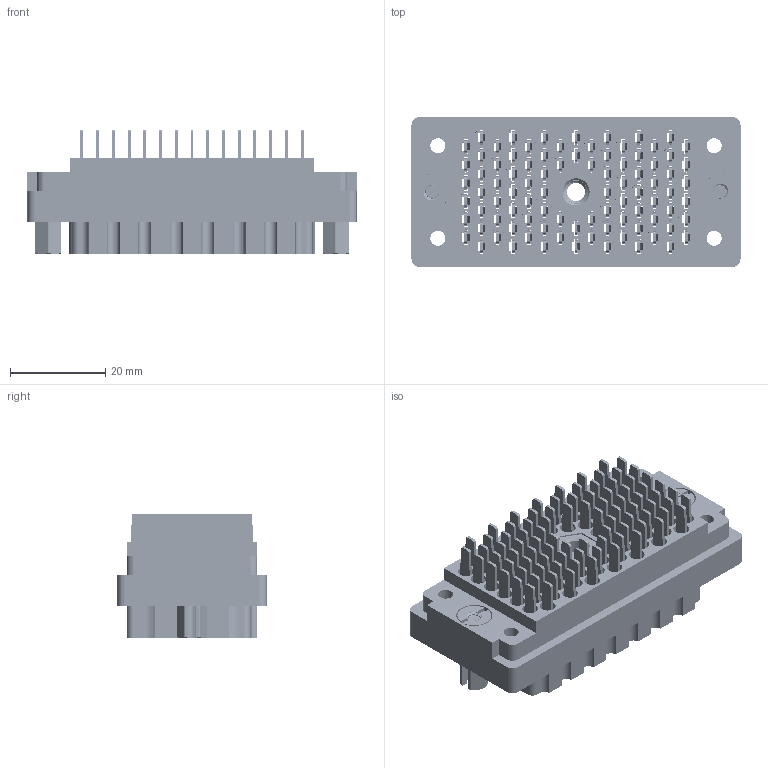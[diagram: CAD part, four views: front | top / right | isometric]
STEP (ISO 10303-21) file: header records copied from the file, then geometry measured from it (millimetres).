
FILE_DESCRIPTION (( 'STEP AP203' ), '1' );
FILE_NAME ('516-090-501-202.STEP', '2020-09-08T17:35:47', ( '' ), ( '' ), 'SwSTEP 2.0', 'SolidWorks 2020', '' );
FILE_SCHEMA (( 'CONFIG_CONTROL_DESIGN' ));
Length unit declared in the file: inch
Products named in the file (7): 516-252-095-100; 516-221-090-102_091; 516-090-501-202; 516-292-001_501 Contact; 516-221-090-102_090; 516-252-091-102; 516 Part Receptacle_090
Assembly tree (97 placements, depth 2):
  516-090-501-202
    516 Part Receptacle_090
    516-292-001_501 Contact  x91
    516-252-091-102  x2
    516-221-090-102_090
    516-252-095-100
    516-221-090-102_091
Bounding box: 69.04 x 31.34 x 26.21 mm (x, y, z)
Volume: 24249.5 mm3; surface area: 48061.7 mm2
Topology: 97 solids, 97 shells, 8683 faces, 25195 edges, 16723 vertices
Faces by surface type: plane 5163, cylinder 2900, bspline 574, cone 46
Entity records: 83650 total; most frequent: CARTESIAN_POINT 20786, ORIENTED_EDGE 12786, DIRECTION 12276, EDGE_CURVE 6393, VECTOR 4538, LINE 4538, VERTEX_POINT 4251, AXIS2_PLACEMENT_3D 3869
